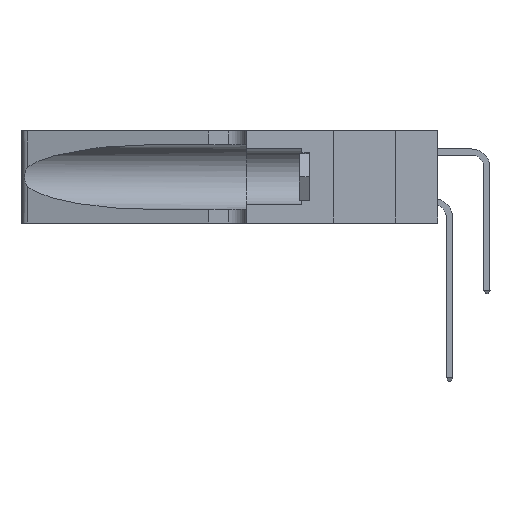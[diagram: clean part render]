
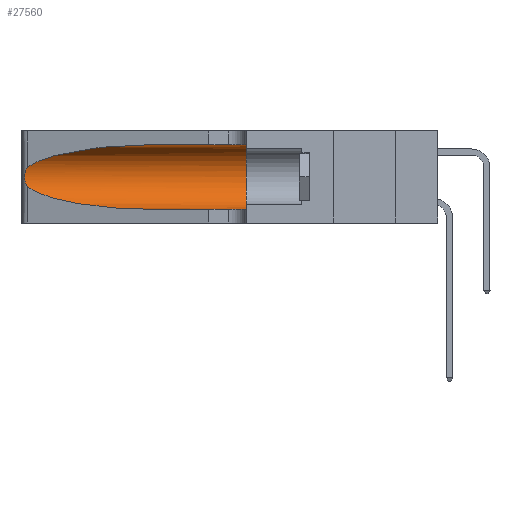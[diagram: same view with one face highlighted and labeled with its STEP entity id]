
A CAD part, left-side view. The second image highlights one B-rep face of the part: STEP entity #27560.
In plain terms, the highlighted cylindrical face has radius 3.308 mm (diameter 6.617 mm), a partial arc.
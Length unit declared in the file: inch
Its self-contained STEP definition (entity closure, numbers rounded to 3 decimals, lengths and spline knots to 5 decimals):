
#337 = CARTESIAN_POINT ( 'NONE',  ( 0.26075, 1.23896, 0.178 ) ) ;
#2305 = DIRECTION ( 'NONE',  ( 0., -1., 0. ) ) ;
#2529 = VERTEX_POINT ( 'NONE', #33349 ) ;
#2861 = CARTESIAN_POINT ( 'NONE',  ( 0.1305, 0.72297, 0.31525 ) ) ;
#3099 = CARTESIAN_POINT ( 'NONE',  ( 0.1305, 0.35, 0.185 ) ) ;
#3115 = ORIENTED_EDGE ( 'NONE', *, *, #29376, .T. ) ;
#3370 = CARTESIAN_POINT ( 'NONE',  ( 0.25555, 1.22993, 0.14849 ) ) ;
#3910 = VERTEX_POINT ( 'NONE', #19078 ) ;
#4260 = ORIENTED_EDGE ( 'NONE', *, *, #7136, .F. ) ;
#6059 = CARTESIAN_POINT ( 'NONE',  ( 0.25856, 1.23593, 0.16098 ) ) ;
#7136 = EDGE_CURVE ( 'NONE', #2529, #16821, #7241, .T. ) ;
#7241 = LINE ( 'NONE', #21507, #11644 ) ;
#7909 = CARTESIAN_POINT ( 'NONE',  ( 0.1305, 1.61858, 0.185 ) ) ;
#9250 = CARTESIAN_POINT ( 'NONE',  ( 0.25487, 1.22718, 0.22369 ) ) ;
#9404 = CARTESIAN_POINT ( 'NONE',  ( 0.1305, 0.72297, 0.05475 ) ) ;
#10080 = EDGE_CURVE ( 'NONE', #16821, #3910, #10574, .T. ) ;
#10574 = CIRCLE ( 'NONE', #29467, 0.13025 ) ;
#11423 = EDGE_LOOP ( 'NONE', ( #25103, #17358, #29440, #3115, #17781, #4260 ) ) ;
#11644 = VECTOR ( 'NONE', #24231, 39.37008 ) ;
#11967 = VERTEX_POINT ( 'NONE', #19433 ) ;
#12287 =( BOUNDED_CURVE ( )  B_SPLINE_CURVE ( 3, ( #20325, #26235, #28805, #9404 ),
 .UNSPECIFIED., .F., .F. ) 
 B_SPLINE_CURVE_WITH_KNOTS ( ( 4, 4 ),
 ( 3.44316, 4.71239 ),
 .UNSPECIFIED. ) 
 CURVE ( )  GEOMETRIC_REPRESENTATION_ITEM ( )  RATIONAL_B_SPLINE_CURVE ( ( 1., 0.87, 0.87, 1. ) ) 
 REPRESENTATION_ITEM ( '' )  );
#14242 = CARTESIAN_POINT ( 'NONE',  ( 0.25789, 1.23486, 0.15765 ) ) ;
#14604 = CARTESIAN_POINT ( 'NONE',  ( 0.26017, 1.23833, 0.17102 ) ) ;
#16026 = CARTESIAN_POINT ( 'NONE',  ( 0.25487, 1.22718, 0.22369 ) ) ;
#16552 = CARTESIAN_POINT ( 'NONE',  ( 0.1305, 0.72297, 0.05475 ) ) ;
#16818 = CARTESIAN_POINT ( 'NONE',  ( 0.18966, 0.96281, 0.31525 ) ) ;
#16821 = VERTEX_POINT ( 'NONE', #31062 ) ;
#17104 = CARTESIAN_POINT ( 'NONE',  ( 0.26018, 1.23835, 0.19895 ) ) ;
#17217 = CARTESIAN_POINT ( 'NONE',  ( 0.25487, 1.22718, 0.14631 ) ) ;
#17335 = CARTESIAN_POINT ( 'NONE',  ( 0.25787, 1.23484, 0.2124 ) ) ;
#17358 = ORIENTED_EDGE ( 'NONE', *, *, #27945, .T. ) ;
#17781 = ORIENTED_EDGE ( 'NONE', *, *, #10080, .F. ) ;
#17952 = CYLINDRICAL_SURFACE ( 'NONE', #28944, 0.13025 ) ;
#18217 = DIRECTION ( 'NONE',  ( 0., -1., 0. ) ) ;
#19078 = CARTESIAN_POINT ( 'NONE',  ( 0.1305, 0.35, 0.05475 ) ) ;
#19433 = CARTESIAN_POINT ( 'NONE',  ( 0.25487, 1.22718, 0.14631 ) ) ;
#19931 = CARTESIAN_POINT ( 'NONE',  ( 0.25639, 1.23186, 0.15144 ) ) ;
#20165 = CARTESIAN_POINT ( 'NONE',  ( 0.25854, 1.2359, 0.20912 ) ) ;
#20275 = CARTESIAN_POINT ( 'NONE',  ( 0.25639, 1.23184, 0.21858 ) ) ;
#20325 = CARTESIAN_POINT ( 'NONE',  ( 0.25487, 1.22718, 0.14631 ) ) ;
#21507 = CARTESIAN_POINT ( 'NONE',  ( 0.1305, 1.61858, 0.31525 ) ) ;
#21768 = B_SPLINE_CURVE_WITH_KNOTS ( 'NONE', 3,
 ( #9250, #28878, #20275, #17335, #20165, #17104, #31223, #337, #14604, #6059, #14242, #19931, #3370, #17217 ),
 .UNSPECIFIED., .F., .F.,
 ( 4, 2, 2, 2, 2, 2, 4 ),
 ( 0., 0.00027, 0.00053, 0.00107, 0.0016, 0.00187, 0.00214 ),
 .UNSPECIFIED. ) ;
#22381 = CARTESIAN_POINT ( 'NONE',  ( 0.2373, 1.15595, 0.28018 ) ) ;
#22489 = VERTEX_POINT ( 'NONE', #16026 ) ;
#23286 = FACE_OUTER_BOUND ( 'NONE', #11423, .T. ) ;
#24231 = DIRECTION ( 'NONE',  ( 0., -1., 0. ) ) ;
#24414 = VERTEX_POINT ( 'NONE', #16552 ) ;
#24969 = CARTESIAN_POINT ( 'NONE',  ( 0.25487, 1.22718, 0.22369 ) ) ;
#25103 = ORIENTED_EDGE ( 'NONE', *, *, #30367, .T. ) ;
#25557 = DIRECTION ( 'NONE',  ( 0., 1., 0. ) ) ;
#26235 = CARTESIAN_POINT ( 'NONE',  ( 0.2373, 1.15595, 0.08982 ) ) ;
#27560 = ADVANCED_FACE ( 'NONE', ( #23286 ), #17952, .F. ) ;
#27945 = EDGE_CURVE ( 'NONE', #22489, #11967, #21768, .T. ) ;
#28364 = DIRECTION ( 'NONE',  ( 0., 0., 1. ) ) ;
#28805 = CARTESIAN_POINT ( 'NONE',  ( 0.18966, 0.96281, 0.05475 ) ) ;
#28878 = CARTESIAN_POINT ( 'NONE',  ( 0.25555, 1.22994, 0.2215 ) ) ;
#28944 = AXIS2_PLACEMENT_3D ( 'NONE', #7909, #2305, #35874 ) ;
#29376 = EDGE_CURVE ( 'NONE', #24414, #3910, #33242, .T. ) ;
#29440 = ORIENTED_EDGE ( 'NONE', *, *, #31099, .T. ) ;
#29467 = AXIS2_PLACEMENT_3D ( 'NONE', #3099, #25557, #28364 ) ;
#30367 = EDGE_CURVE ( 'NONE', #2529, #22489, #31884, .T. ) ;
#31062 = CARTESIAN_POINT ( 'NONE',  ( 0.1305, 0.35, 0.31525 ) ) ;
#31099 = EDGE_CURVE ( 'NONE', #11967, #24414, #12287, .T. ) ;
#31223 = CARTESIAN_POINT ( 'NONE',  ( 0.26075, 1.23896, 0.19203 ) ) ;
#31494 = VECTOR ( 'NONE', #18217, 39.37008 ) ;
#31884 =( BOUNDED_CURVE ( )  B_SPLINE_CURVE ( 3, ( #2861, #16818, #22381, #24969 ),
 .UNSPECIFIED., .F., .F. ) 
 B_SPLINE_CURVE_WITH_KNOTS ( ( 4, 4 ),
 ( 1.5708, 2.84003 ),
 .UNSPECIFIED. ) 
 CURVE ( )  GEOMETRIC_REPRESENTATION_ITEM ( )  RATIONAL_B_SPLINE_CURVE ( ( 1., 0.87, 0.87, 1. ) ) 
 REPRESENTATION_ITEM ( '' )  );
#33242 = LINE ( 'NONE', #34799, #31494 ) ;
#33349 = CARTESIAN_POINT ( 'NONE',  ( 0.1305, 0.72297, 0.31525 ) ) ;
#34799 = CARTESIAN_POINT ( 'NONE',  ( 0.1305, 1.61858, 0.05475 ) ) ;
#35874 = DIRECTION ( 'NONE',  ( 0., 0., -1. ) ) ;
